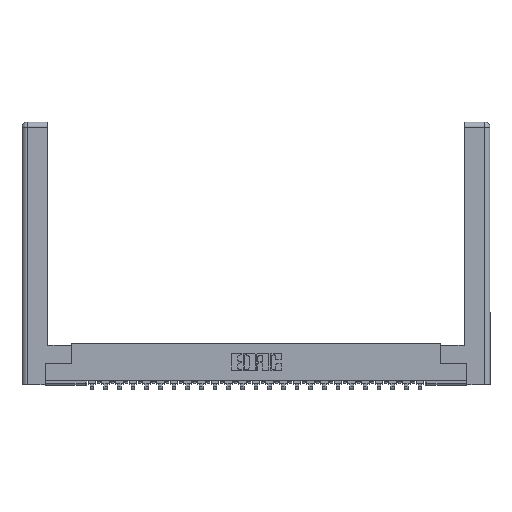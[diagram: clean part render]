
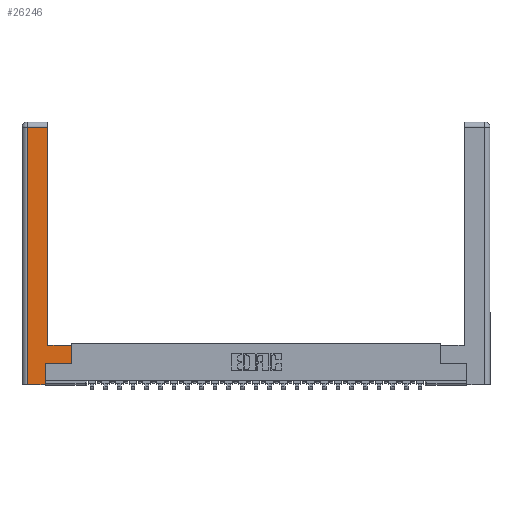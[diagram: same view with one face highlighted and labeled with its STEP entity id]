
A CAD part, top view. The second image highlights one B-rep face of the part: STEP entity #26246.
In plain terms, the highlighted planar face has unit normal (0, 0, 1).
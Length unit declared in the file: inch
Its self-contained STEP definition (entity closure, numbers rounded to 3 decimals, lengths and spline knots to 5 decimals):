
#24 = CARTESIAN_POINT ( 'NONE',  ( 0.0615, 0., 0. ) ) ;
#387 = PLANE ( 'NONE',  #23526 ) ;
#683 = LINE ( 'NONE', #21721, #22197 ) ;
#685 = EDGE_CURVE ( 'NONE', #14263, #20959, #24488, .T. ) ;
#860 = CARTESIAN_POINT ( 'NONE',  ( 0.295, 0.45, 0. ) ) ;
#1012 = ORIENTED_EDGE ( 'NONE', *, *, #685, .T. ) ;
#1195 = ORIENTED_EDGE ( 'NONE', *, *, #24934, .T. ) ;
#2213 = ORIENTED_EDGE ( 'NONE', *, *, #3910, .T. ) ;
#2978 = VERTEX_POINT ( 'NONE', #7612 ) ;
#3695 = CARTESIAN_POINT ( 'NONE',  ( 0.565, 0.45, 0. ) ) ;
#3733 = DIRECTION ( 'NONE',  ( 0., 1., 0. ) ) ;
#3910 = EDGE_CURVE ( 'NONE', #2978, #12956, #15790, .T. ) ;
#3970 = LINE ( 'NONE', #13694, #17184 ) ;
#4129 = DIRECTION ( 'NONE',  ( 0., -1., 0. ) ) ;
#4340 = VERTEX_POINT ( 'NONE', #3695 ) ;
#4564 = DIRECTION ( 'NONE',  ( -1., 0., 0. ) ) ;
#4594 = VERTEX_POINT ( 'NONE', #9525 ) ;
#5233 = DIRECTION ( 'NONE',  ( -1., 0., 0. ) ) ;
#5389 = VECTOR ( 'NONE', #22059, 39.37008 ) ;
#5639 = EDGE_CURVE ( 'NONE', #24297, #2978, #3970, .T. ) ;
#6472 = DIRECTION ( 'NONE',  ( 0., 0., -1. ) ) ;
#6734 = CARTESIAN_POINT ( 'NONE',  ( 0., 0., 0. ) ) ;
#6814 = DIRECTION ( 'NONE',  ( -1., 0., 0. ) ) ;
#7612 = CARTESIAN_POINT ( 'NONE',  ( 0.265, 0.245, 0. ) ) ;
#7913 = CARTESIAN_POINT ( 'NONE',  ( 0.0615, 2.94, 0. ) ) ;
#8088 = VECTOR ( 'NONE', #14585, 39.37008 ) ;
#8552 = ORIENTED_EDGE ( 'NONE', *, *, #17378, .T. ) ;
#8703 = LINE ( 'NONE', #16696, #8088 ) ;
#9494 = FACE_OUTER_BOUND ( 'NONE', #15894, .T. ) ;
#9525 = CARTESIAN_POINT ( 'NONE',  ( 0.0615, 0., 0. ) ) ;
#9587 = DIRECTION ( 'NONE',  ( 1., 0., 0. ) ) ;
#9819 = VERTEX_POINT ( 'NONE', #860 ) ;
#10878 = LINE ( 'NONE', #11913, #5389 ) ;
#10953 = DIRECTION ( 'NONE',  ( 0., 1., 0. ) ) ;
#11848 = CARTESIAN_POINT ( 'NONE',  ( 0.565, 0.245, 0. ) ) ;
#11879 = VECTOR ( 'NONE', #9587, 39.37008 ) ;
#11913 = CARTESIAN_POINT ( 'NONE',  ( 0.265, 0., 0. ) ) ;
#12680 = EDGE_CURVE ( 'NONE', #12956, #4340, #15093, .T. ) ;
#12879 = CARTESIAN_POINT ( 'NONE',  ( 0.0615, 2.94, 0. ) ) ;
#12956 = VERTEX_POINT ( 'NONE', #22645 ) ;
#12962 = CARTESIAN_POINT ( 'NONE',  ( 0.295, 2.94, 0. ) ) ;
#13501 = VECTOR ( 'NONE', #3733, 39.37008 ) ;
#13694 = CARTESIAN_POINT ( 'NONE',  ( 0.265, 0.245, 0. ) ) ;
#14263 = VERTEX_POINT ( 'NONE', #12962 ) ;
#14585 = DIRECTION ( 'NONE',  ( 0., 1., 0. ) ) ;
#15093 = LINE ( 'NONE', #17865, #13501 ) ;
#15790 = LINE ( 'NONE', #11848, #11879 ) ;
#15799 = EDGE_CURVE ( 'NONE', #4340, #9819, #683, .T. ) ;
#15894 = EDGE_LOOP ( 'NONE', ( #8552, #1012, #1195, #24413, #16297, #2213, #18259, #23673 ) ) ;
#16297 = ORIENTED_EDGE ( 'NONE', *, *, #5639, .T. ) ;
#16421 = CARTESIAN_POINT ( 'NONE',  ( 0.265, 0., 0. ) ) ;
#16696 = CARTESIAN_POINT ( 'NONE',  ( 0.295, 3., 0. ) ) ;
#16922 = VECTOR ( 'NONE', #6814, 39.37008 ) ;
#17184 = VECTOR ( 'NONE', #10953, 39.37008 ) ;
#17378 = EDGE_CURVE ( 'NONE', #9819, #14263, #8703, .T. ) ;
#17865 = CARTESIAN_POINT ( 'NONE',  ( 0.565, 0.45, 0. ) ) ;
#18259 = ORIENTED_EDGE ( 'NONE', *, *, #12680, .T. ) ;
#20959 = VERTEX_POINT ( 'NONE', #7913 ) ;
#21651 = VECTOR ( 'NONE', #4129, 39.37008 ) ;
#21721 = CARTESIAN_POINT ( 'NONE',  ( 0.295, 0.45, 0. ) ) ;
#22059 = DIRECTION ( 'NONE',  ( 1., 0., 0. ) ) ;
#22197 = VECTOR ( 'NONE', #5233, 39.37008 ) ;
#22636 = LINE ( 'NONE', #24, #21651 ) ;
#22645 = CARTESIAN_POINT ( 'NONE',  ( 0.565, 0.245, 0. ) ) ;
#23526 = AXIS2_PLACEMENT_3D ( 'NONE', #6734, #6472, #4564 ) ;
#23673 = ORIENTED_EDGE ( 'NONE', *, *, #15799, .T. ) ;
#24297 = VERTEX_POINT ( 'NONE', #16421 ) ;
#24413 = ORIENTED_EDGE ( 'NONE', *, *, #24734, .T. ) ;
#24488 = LINE ( 'NONE', #12879, #16922 ) ;
#24734 = EDGE_CURVE ( 'NONE', #4594, #24297, #10878, .T. ) ;
#24934 = EDGE_CURVE ( 'NONE', #20959, #4594, #22636, .T. ) ;
#26246 = ADVANCED_FACE ( 'NONE', ( #9494 ), #387, .F. ) ;
